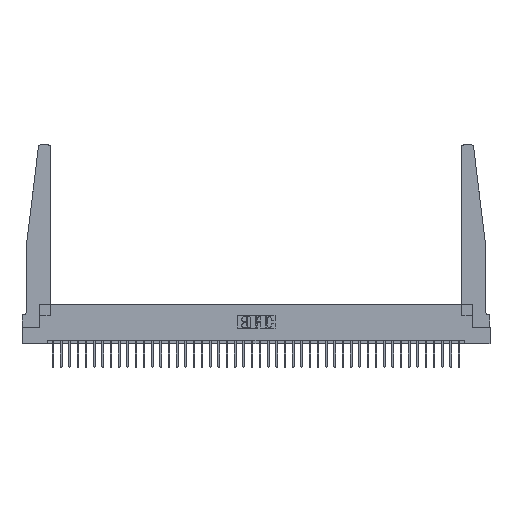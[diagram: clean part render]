
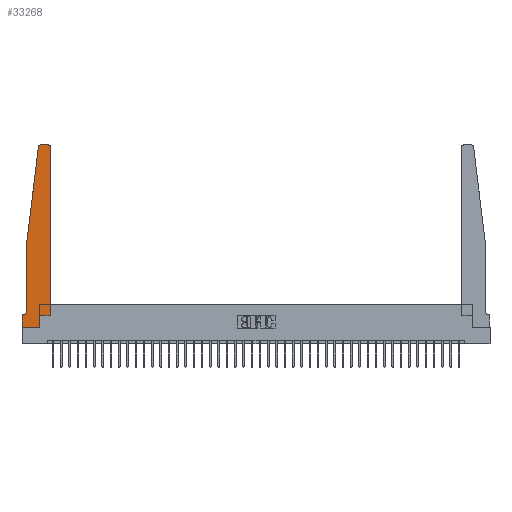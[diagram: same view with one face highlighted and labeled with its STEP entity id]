
A CAD part, top view. The second image highlights one B-rep face of the part: STEP entity #33268.
In plain terms, the highlighted planar face has unit normal (0, 0, 1).
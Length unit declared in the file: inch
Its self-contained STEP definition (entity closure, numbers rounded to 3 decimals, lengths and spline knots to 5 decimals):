
#39 = EDGE_CURVE ( 'NONE', #8069, #29596, #24533, .T. ) ;
#195 = VECTOR ( 'NONE', #4748, 39.37008 ) ;
#1007 = DIRECTION ( 'NONE',  ( 0., 0., 1. ) ) ;
#2143 = CARTESIAN_POINT ( 'NONE',  ( 0.065, 1.25, 0.37 ) ) ;
#2774 = DIRECTION ( 'NONE',  ( 1., 0., 0. ) ) ;
#3147 = DIRECTION ( 'NONE',  ( -1., 0., 0. ) ) ;
#3180 = DIRECTION ( 'NONE',  ( 0., 1., 0. ) ) ;
#4173 = EDGE_CURVE ( 'NONE', #19396, #11997, #25983, .T. ) ;
#4567 = VECTOR ( 'NONE', #12263, 39.37008 ) ;
#4748 = DIRECTION ( 'NONE',  ( -0.122, -0.992, 0. ) ) ;
#5749 = AXIS2_PLACEMENT_3D ( 'NONE', #25815, #34292, #6155 ) ;
#6050 = AXIS2_PLACEMENT_3D ( 'NONE', #9531, #1007, #20670 ) ;
#6155 = DIRECTION ( 'NONE',  ( -1., 0., 0. ) ) ;
#6219 = CARTESIAN_POINT ( 'NONE',  ( 0.25, 2.75, 0.37 ) ) ;
#6541 = EDGE_CURVE ( 'NONE', #28342, #21073, #9203, .T. ) ;
#6721 = EDGE_CURVE ( 'NONE', #21073, #32384, #15786, .T. ) ;
#7598 = AXIS2_PLACEMENT_3D ( 'NONE', #19138, #36030, #30389 ) ;
#7920 = CARTESIAN_POINT ( 'NONE',  ( 0.425, 2.72, 0.37 ) ) ;
#8069 = VERTEX_POINT ( 'NONE', #25268 ) ;
#8261 = CARTESIAN_POINT ( 'NONE',  ( 0., 0.1875, 0.37 ) ) ;
#8636 = LINE ( 'NONE', #13034, #195 ) ;
#9203 = LINE ( 'NONE', #2143, #10504 ) ;
#9291 = EDGE_CURVE ( 'NONE', #11990, #28342, #8636, .T. ) ;
#9531 = CARTESIAN_POINT ( 'NONE',  ( 0.27653, 2.72, 0.37 ) ) ;
#9640 = CARTESIAN_POINT ( 'NONE',  ( 0.015, 0.1875, 0.37 ) ) ;
#9888 = LINE ( 'NONE', #22054, #31369 ) ;
#10504 = VECTOR ( 'NONE', #21807, 39.37008 ) ;
#11642 = CARTESIAN_POINT ( 'NONE',  ( 0.065, 0.2375, 0.37 ) ) ;
#11990 = VERTEX_POINT ( 'NONE', #15244 ) ;
#11997 = VERTEX_POINT ( 'NONE', #31990 ) ;
#12263 = DIRECTION ( 'NONE',  ( 0., 1., 0. ) ) ;
#12309 = LINE ( 'NONE', #6219, #23706 ) ;
#12621 = EDGE_CURVE ( 'NONE', #17325, #26127, #27922, .T. ) ;
#12648 = ORIENTED_EDGE ( 'NONE', *, *, #18350, .T. ) ;
#13034 = CARTESIAN_POINT ( 'NONE',  ( 0.065, 1.25, 0.37 ) ) ;
#13119 = CARTESIAN_POINT ( 'NONE',  ( 0.065, 0.1875, 0.37 ) ) ;
#13881 = LINE ( 'NONE', #29047, #4567 ) ;
#14492 = CARTESIAN_POINT ( 'NONE',  ( 0.395, 2.75, 0.37 ) ) ;
#14921 = VECTOR ( 'NONE', #27307, 39.37008 ) ;
#15244 = CARTESIAN_POINT ( 'NONE',  ( 0.24675, 2.72367, 0.37 ) ) ;
#15647 = ORIENTED_EDGE ( 'NONE', *, *, #25704, .T. ) ;
#15786 = CIRCLE ( 'NONE', #5749, 0.05 ) ;
#16330 = LINE ( 'NONE', #20042, #21990 ) ;
#16492 = EDGE_CURVE ( 'NONE', #11997, #17325, #16330, .T. ) ;
#16619 = DIRECTION ( 'NONE',  ( 0., 0., 1. ) ) ;
#17325 = VERTEX_POINT ( 'NONE', #7920 ) ;
#17564 = ORIENTED_EDGE ( 'NONE', *, *, #35447, .T. ) ;
#17797 = VECTOR ( 'NONE', #19022, 39.37008 ) ;
#17847 = CARTESIAN_POINT ( 'NONE',  ( 0.2605, 0., 0.37 ) ) ;
#18001 = VERTEX_POINT ( 'NONE', #31820 ) ;
#18154 = CARTESIAN_POINT ( 'NONE',  ( 0.2605, 0.18, 0.37 ) ) ;
#18350 = EDGE_CURVE ( 'NONE', #32384, #18001, #25222, .T. ) ;
#18814 = AXIS2_PLACEMENT_3D ( 'NONE', #8261, #16619, #2774 ) ;
#19022 = DIRECTION ( 'NONE',  ( -1., 0., 0. ) ) ;
#19138 = CARTESIAN_POINT ( 'NONE',  ( 0.395, 2.72, 0.37 ) ) ;
#19396 = VERTEX_POINT ( 'NONE', #18154 ) ;
#20042 = CARTESIAN_POINT ( 'NONE',  ( 0.425, 0.18, 0.37 ) ) ;
#20274 = ORIENTED_EDGE ( 'NONE', *, *, #30930, .T. ) ;
#20670 = DIRECTION ( 'NONE',  ( 1., 0., 0. ) ) ;
#20686 = ORIENTED_EDGE ( 'NONE', *, *, #16492, .T. ) ;
#20765 = DIRECTION ( 'NONE',  ( 1., 0., 0. ) ) ;
#21073 = VERTEX_POINT ( 'NONE', #11642 ) ;
#21504 = ORIENTED_EDGE ( 'NONE', *, *, #39, .T. ) ;
#21807 = DIRECTION ( 'NONE',  ( 0., -1., 0. ) ) ;
#21990 = VECTOR ( 'NONE', #3180, 39.37008 ) ;
#22054 = CARTESIAN_POINT ( 'NONE',  ( 0., 0., 0.37 ) ) ;
#22078 = ORIENTED_EDGE ( 'NONE', *, *, #35042, .T. ) ;
#22687 = ORIENTED_EDGE ( 'NONE', *, *, #4173, .T. ) ;
#23706 = VECTOR ( 'NONE', #3147, 39.37008 ) ;
#23942 = ORIENTED_EDGE ( 'NONE', *, *, #12621, .T. ) ;
#24533 = LINE ( 'NONE', #27677, #14921 ) ;
#24675 = VERTEX_POINT ( 'NONE', #35832 ) ;
#24873 = DIRECTION ( 'NONE',  ( 0., -1., 0. ) ) ;
#25222 = LINE ( 'NONE', #13119, #17797 ) ;
#25268 = CARTESIAN_POINT ( 'NONE',  ( 0., 0., 0.37 ) ) ;
#25704 = EDGE_CURVE ( 'NONE', #29596, #19396, #13881, .T. ) ;
#25815 = CARTESIAN_POINT ( 'NONE',  ( 0.015, 0.2375, 0.37 ) ) ;
#25983 = LINE ( 'NONE', #29089, #28220 ) ;
#26127 = VERTEX_POINT ( 'NONE', #14492 ) ;
#27307 = DIRECTION ( 'NONE',  ( 1., 0., 0. ) ) ;
#27677 = CARTESIAN_POINT ( 'NONE',  ( 0., 0., 0.37 ) ) ;
#27922 = CIRCLE ( 'NONE', #7598, 0.03 ) ;
#28220 = VECTOR ( 'NONE', #20765, 39.37008 ) ;
#28320 = ORIENTED_EDGE ( 'NONE', *, *, #9291, .T. ) ;
#28342 = VERTEX_POINT ( 'NONE', #32872 ) ;
#29047 = CARTESIAN_POINT ( 'NONE',  ( 0.2605, 0.18, 0.37 ) ) ;
#29089 = CARTESIAN_POINT ( 'NONE',  ( 0.425, 0.18, 0.37 ) ) ;
#29596 = VERTEX_POINT ( 'NONE', #17847 ) ;
#30037 = ORIENTED_EDGE ( 'NONE', *, *, #6541, .T. ) ;
#30389 = DIRECTION ( 'NONE',  ( 1., 0., 0. ) ) ;
#30575 = PLANE ( 'NONE',  #18814 ) ;
#30930 = EDGE_CURVE ( 'NONE', #26127, #24675, #12309, .T. ) ;
#31369 = VECTOR ( 'NONE', #24873, 39.37008 ) ;
#31820 = CARTESIAN_POINT ( 'NONE',  ( 0., 0.1875, 0.37 ) ) ;
#31990 = CARTESIAN_POINT ( 'NONE',  ( 0.425, 0.18, 0.37 ) ) ;
#32380 = ORIENTED_EDGE ( 'NONE', *, *, #6721, .T. ) ;
#32384 = VERTEX_POINT ( 'NONE', #9640 ) ;
#32794 = FACE_OUTER_BOUND ( 'NONE', #34070, .T. ) ;
#32872 = CARTESIAN_POINT ( 'NONE',  ( 0.065, 1.25, 0.37 ) ) ;
#33268 = ADVANCED_FACE ( 'NONE', ( #32794 ), #30575, .T. ) ;
#34070 = EDGE_LOOP ( 'NONE', ( #20274, #17564, #28320, #30037, #32380, #12648, #22078, #21504, #15647, #22687, #20686, #23942 ) ) ;
#34292 = DIRECTION ( 'NONE',  ( 0., 0., -1. ) ) ;
#35042 = EDGE_CURVE ( 'NONE', #18001, #8069, #9888, .T. ) ;
#35447 = EDGE_CURVE ( 'NONE', #24675, #11990, #36171, .T. ) ;
#35832 = CARTESIAN_POINT ( 'NONE',  ( 0.27653, 2.75, 0.37 ) ) ;
#36030 = DIRECTION ( 'NONE',  ( 0., 0., 1. ) ) ;
#36171 = CIRCLE ( 'NONE', #6050, 0.03 ) ;
